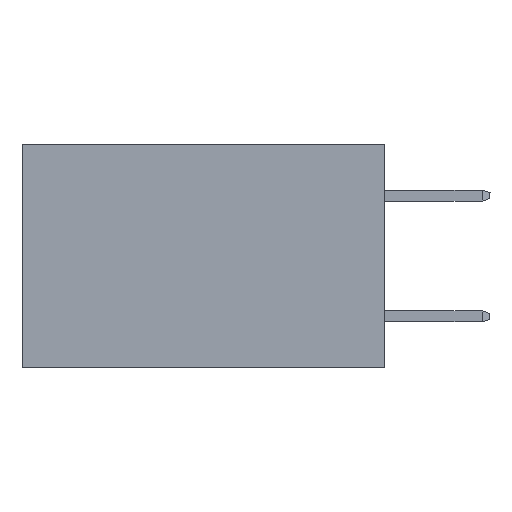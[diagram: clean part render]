
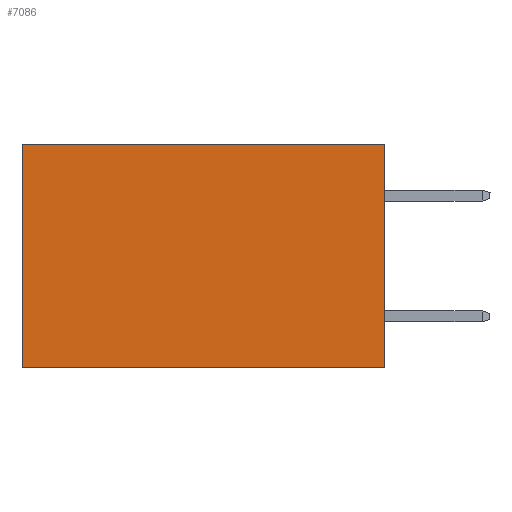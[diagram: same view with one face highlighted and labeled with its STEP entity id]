
A CAD part, left-side view. The second image highlights one B-rep face of the part: STEP entity #7086.
In plain terms, the highlighted planar face has unit normal (-1, 0, 0).
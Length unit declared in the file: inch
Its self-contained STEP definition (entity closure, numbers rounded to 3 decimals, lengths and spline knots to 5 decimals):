
#1262 = CARTESIAN_POINT ( 'NONE',  ( 0.2615, 0., -0.37 ) ) ;
#1561 = AXIS2_PLACEMENT_3D ( 'NONE', #14036, #1750, #16001 ) ;
#1645 = VECTOR ( 'NONE', #19636, 39.37008 ) ;
#1750 = DIRECTION ( 'NONE',  ( 1., 0., 0. ) ) ;
#1924 = CARTESIAN_POINT ( 'NONE',  ( 0.2615, 0.6, 0. ) ) ;
#2302 = LINE ( 'NONE', #1262, #1645 ) ;
#3094 = CARTESIAN_POINT ( 'NONE',  ( 0.2615, 0., 0. ) ) ;
#4592 = EDGE_CURVE ( 'NONE', #14429, #23738, #20749, .T. ) ;
#4917 = EDGE_CURVE ( 'NONE', #18226, #8721, #21393, .T. ) ;
#4953 = EDGE_CURVE ( 'NONE', #14429, #18226, #26078, .T. ) ;
#5264 = VECTOR ( 'NONE', #11262, 39.37008 ) ;
#5882 = PLANE ( 'NONE',  #1561 ) ;
#7086 = ADVANCED_FACE ( 'NONE', ( #9662 ), #5882, .F. ) ;
#8721 = VERTEX_POINT ( 'NONE', #20625 ) ;
#9662 = FACE_OUTER_BOUND ( 'NONE', #21436, .T. ) ;
#9895 = DIRECTION ( 'NONE',  ( 0., 1., 0. ) ) ;
#10174 = CARTESIAN_POINT ( 'NONE',  ( 0.2615, 0., 0. ) ) ;
#11262 = DIRECTION ( 'NONE',  ( 0., 0., -1. ) ) ;
#11300 = CARTESIAN_POINT ( 'NONE',  ( 0.2615, 0.6, -0.37 ) ) ;
#11307 = EDGE_CURVE ( 'NONE', #23738, #8721, #2302, .T. ) ;
#12656 = ORIENTED_EDGE ( 'NONE', *, *, #11307, .F. ) ;
#14036 = CARTESIAN_POINT ( 'NONE',  ( 0.2615, 0., -0.37 ) ) ;
#14429 = VERTEX_POINT ( 'NONE', #3094 ) ;
#14756 = VECTOR ( 'NONE', #20372, 39.37008 ) ;
#15999 = VECTOR ( 'NONE', #9895, 39.37008 ) ;
#16001 = DIRECTION ( 'NONE',  ( 0., 0., -1. ) ) ;
#18226 = VERTEX_POINT ( 'NONE', #1924 ) ;
#18573 = ORIENTED_EDGE ( 'NONE', *, *, #4953, .T. ) ;
#19199 = ORIENTED_EDGE ( 'NONE', *, *, #4592, .F. ) ;
#19636 = DIRECTION ( 'NONE',  ( 0., 1., 0. ) ) ;
#20372 = DIRECTION ( 'NONE',  ( 0., 0., -1. ) ) ;
#20432 = CARTESIAN_POINT ( 'NONE',  ( 0.2615, 0., -0.37 ) ) ;
#20625 = CARTESIAN_POINT ( 'NONE',  ( 0.2615, 0.6, -0.37 ) ) ;
#20749 = LINE ( 'NONE', #20432, #14756 ) ;
#21393 = LINE ( 'NONE', #11300, #5264 ) ;
#21436 = EDGE_LOOP ( 'NONE', ( #25417, #12656, #19199, #18573 ) ) ;
#22486 = CARTESIAN_POINT ( 'NONE',  ( 0.2615, 0., -0.37 ) ) ;
#23738 = VERTEX_POINT ( 'NONE', #22486 ) ;
#25417 = ORIENTED_EDGE ( 'NONE', *, *, #4917, .T. ) ;
#26078 = LINE ( 'NONE', #10174, #15999 ) ;
